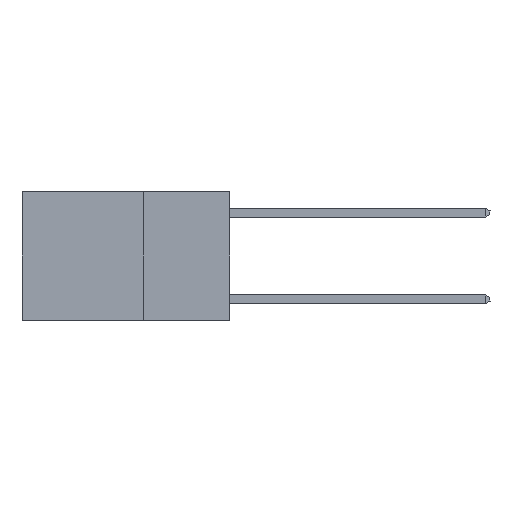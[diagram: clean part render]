
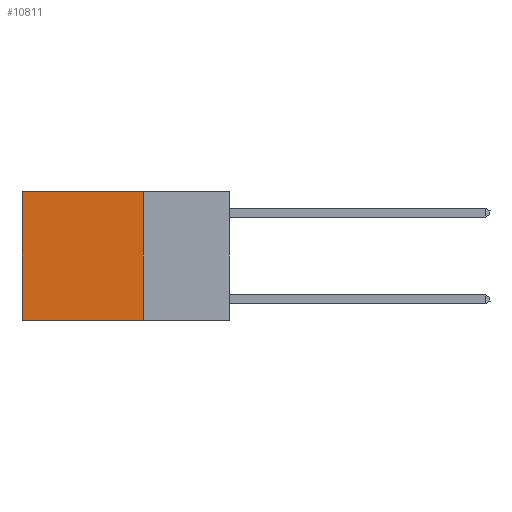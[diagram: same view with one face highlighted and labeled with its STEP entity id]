
A CAD part, left-side view. The second image highlights one B-rep face of the part: STEP entity #10811.
In plain terms, the highlighted planar face has unit normal (-1, 0, 0).
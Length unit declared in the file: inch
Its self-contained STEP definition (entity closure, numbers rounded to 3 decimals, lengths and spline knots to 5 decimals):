
#28 = VERTEX_POINT ( 'NONE', #12550 ) ;
#134 = EDGE_CURVE ( 'NONE', #28, #1787, #11738, .T. ) ;
#899 = CARTESIAN_POINT ( 'NONE',  ( 0.2625, 0.25, 0. ) ) ;
#1787 = VERTEX_POINT ( 'NONE', #12575 ) ;
#1820 = DIRECTION ( 'NONE',  ( 0., 1., 0. ) ) ;
#1898 = CARTESIAN_POINT ( 'NONE',  ( 0.2625, 0.25, 0. ) ) ;
#3027 = LINE ( 'NONE', #3166, #3386 ) ;
#3166 = CARTESIAN_POINT ( 'NONE',  ( 0.2625, 0.25, 0. ) ) ;
#3386 = VECTOR ( 'NONE', #8206, 39.37008 ) ;
#3464 = LINE ( 'NONE', #12443, #6348 ) ;
#3640 = VECTOR ( 'NONE', #1820, 39.37008 ) ;
#3698 = CARTESIAN_POINT ( 'NONE',  ( 0.2625, 0.6, 0. ) ) ;
#4276 = ORIENTED_EDGE ( 'NONE', *, *, #134, .F. ) ;
#4997 = DIRECTION ( 'NONE',  ( 0., 0., -1. ) ) ;
#5666 = CARTESIAN_POINT ( 'NONE',  ( 0.2625, 0.25, -0.37 ) ) ;
#5780 = VECTOR ( 'NONE', #5843, 39.37008 ) ;
#5843 = DIRECTION ( 'NONE',  ( 0., 1., 0. ) ) ;
#5914 = FACE_OUTER_BOUND ( 'NONE', #11415, .T. ) ;
#6348 = VECTOR ( 'NONE', #8248, 39.37008 ) ;
#6920 = VERTEX_POINT ( 'NONE', #9846 ) ;
#7013 = ORIENTED_EDGE ( 'NONE', *, *, #10810, .T. ) ;
#7722 = EDGE_CURVE ( 'NONE', #10475, #1787, #3464, .T. ) ;
#8206 = DIRECTION ( 'NONE',  ( 0., 0., -1. ) ) ;
#8248 = DIRECTION ( 'NONE',  ( 0., 0., -1. ) ) ;
#8384 = ORIENTED_EDGE ( 'NONE', *, *, #9447, .F. ) ;
#9447 = EDGE_CURVE ( 'NONE', #6920, #28, #3027, .T. ) ;
#9846 = CARTESIAN_POINT ( 'NONE',  ( 0.2625, 0.25, 0. ) ) ;
#10029 = PLANE ( 'NONE',  #11028 ) ;
#10475 = VERTEX_POINT ( 'NONE', #3698 ) ;
#10810 = EDGE_CURVE ( 'NONE', #6920, #10475, #10943, .T. ) ;
#10811 = ADVANCED_FACE ( 'NONE', ( #5914 ), #10029, .F. ) ;
#10943 = LINE ( 'NONE', #1898, #3640 ) ;
#11028 = AXIS2_PLACEMENT_3D ( 'NONE', #899, #11083, #4997 ) ;
#11083 = DIRECTION ( 'NONE',  ( 1., 0., 0. ) ) ;
#11415 = EDGE_LOOP ( 'NONE', ( #12059, #4276, #8384, #7013 ) ) ;
#11738 = LINE ( 'NONE', #5666, #5780 ) ;
#12059 = ORIENTED_EDGE ( 'NONE', *, *, #7722, .T. ) ;
#12443 = CARTESIAN_POINT ( 'NONE',  ( 0.2625, 0.6, 0. ) ) ;
#12550 = CARTESIAN_POINT ( 'NONE',  ( 0.2625, 0.25, -0.37 ) ) ;
#12575 = CARTESIAN_POINT ( 'NONE',  ( 0.2625, 0.6, -0.37 ) ) ;
